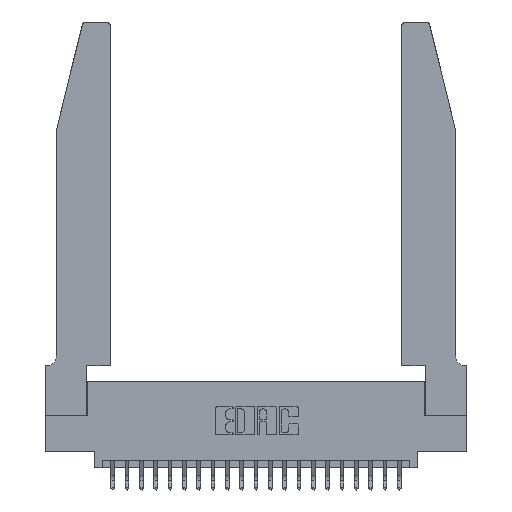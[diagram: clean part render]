
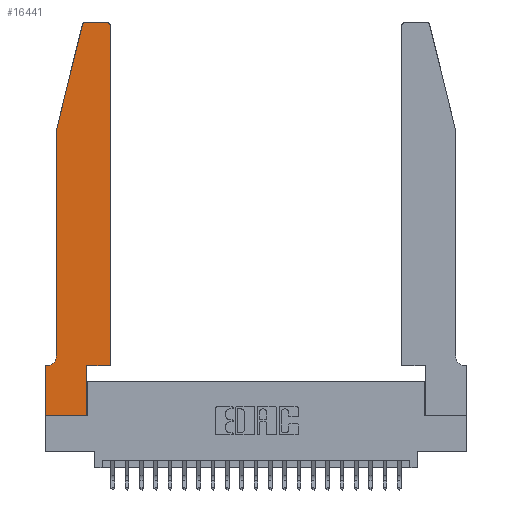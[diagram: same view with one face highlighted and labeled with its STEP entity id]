
A CAD part, top view. The second image highlights one B-rep face of the part: STEP entity #16441.
In plain terms, the highlighted planar face has unit normal (0, 0, 1).
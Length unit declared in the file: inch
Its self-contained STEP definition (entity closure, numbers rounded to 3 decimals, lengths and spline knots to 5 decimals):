
#87 = ORIENTED_EDGE ( 'NONE', *, *, #11937, .T. ) ;
#401 = CARTESIAN_POINT ( 'NONE',  ( 0.0755, 0.42, 0.37 ) ) ;
#807 = CARTESIAN_POINT ( 'NONE',  ( 0.4505, 2.72, 0.37 ) ) ;
#1071 = LINE ( 'NONE', #3253, #11936 ) ;
#1876 = EDGE_CURVE ( 'NONE', #4706, #23011, #15850, .T. ) ;
#1923 = LINE ( 'NONE', #15520, #8670 ) ;
#2167 = AXIS2_PLACEMENT_3D ( 'NONE', #2648, #19357, #4566 ) ;
#2179 = VECTOR ( 'NONE', #7909, 39.37008 ) ;
#2448 = VERTEX_POINT ( 'NONE', #6732 ) ;
#2648 = CARTESIAN_POINT ( 'NONE',  ( 0.284, 2.72, 0.37 ) ) ;
#3219 = CARTESIAN_POINT ( 'NONE',  ( 0.2865, 0.35, 0.37 ) ) ;
#3253 = CARTESIAN_POINT ( 'NONE',  ( 0.0755, 2., 0.37 ) ) ;
#3387 = ORIENTED_EDGE ( 'NONE', *, *, #3504, .T. ) ;
#3462 = CARTESIAN_POINT ( 'NONE',  ( 0., 0., 0.37 ) ) ;
#3504 = EDGE_CURVE ( 'NONE', #12758, #23851, #1071, .T. ) ;
#3602 = EDGE_CURVE ( 'NONE', #20908, #17066, #10462, .T. ) ;
#3861 = ORIENTED_EDGE ( 'NONE', *, *, #23042, .T. ) ;
#4566 = DIRECTION ( 'NONE',  ( 1., 0., 0. ) ) ;
#4706 = VERTEX_POINT ( 'NONE', #401 ) ;
#4806 = ORIENTED_EDGE ( 'NONE', *, *, #15787, .T. ) ;
#4998 = AXIS2_PLACEMENT_3D ( 'NONE', #20359, #10684, #22091 ) ;
#5570 = DIRECTION ( 'NONE',  ( 1., 0., 0. ) ) ;
#6584 = DIRECTION ( 'NONE',  ( -1., 0., 0. ) ) ;
#6600 = ORIENTED_EDGE ( 'NONE', *, *, #14183, .T. ) ;
#6732 = CARTESIAN_POINT ( 'NONE',  ( 0.2865, 0., 0.37 ) ) ;
#6839 = PLANE ( 'NONE',  #19540 ) ;
#6850 = DIRECTION ( 'NONE',  ( -0.239, -0.971, 0. ) ) ;
#6974 = EDGE_CURVE ( 'NONE', #17066, #8709, #1923, .T. ) ;
#7182 = FACE_OUTER_BOUND ( 'NONE', #18135, .T. ) ;
#7399 = DIRECTION ( 'NONE',  ( 1., 0., 0. ) ) ;
#7444 = ORIENTED_EDGE ( 'NONE', *, *, #20225, .T. ) ;
#7909 = DIRECTION ( 'NONE',  ( 0., -1., 0. ) ) ;
#8388 = LINE ( 'NONE', #22264, #13998 ) ;
#8462 = DIRECTION ( 'NONE',  ( 1., 0., 0. ) ) ;
#8602 = CARTESIAN_POINT ( 'NONE',  ( 0.2605, 2.75, 0.37 ) ) ;
#8670 = VECTOR ( 'NONE', #21132, 39.37008 ) ;
#8709 = VERTEX_POINT ( 'NONE', #807 ) ;
#8790 = ORIENTED_EDGE ( 'NONE', *, *, #3602, .T. ) ;
#8804 = LINE ( 'NONE', #15657, #22958 ) ;
#9231 = CARTESIAN_POINT ( 'NONE',  ( 0.25487, 2.72718, 0.37 ) ) ;
#9727 = CARTESIAN_POINT ( 'NONE',  ( 0., 0., 0.37 ) ) ;
#10190 = AXIS2_PLACEMENT_3D ( 'NONE', #14764, #15012, #5570 ) ;
#10255 = CARTESIAN_POINT ( 'NONE',  ( 0.0755, 0.35, 0.37 ) ) ;
#10462 = LINE ( 'NONE', #16329, #13725 ) ;
#10506 = CIRCLE ( 'NONE', #2167, 0.03 ) ;
#10563 = VERTEX_POINT ( 'NONE', #9727 ) ;
#10589 = CARTESIAN_POINT ( 'NONE',  ( 0., 0.35, 0.37 ) ) ;
#10609 = VECTOR ( 'NONE', #16385, 39.37008 ) ;
#10684 = DIRECTION ( 'NONE',  ( 0., 0., -1. ) ) ;
#10894 = LINE ( 'NONE', #3462, #10609 ) ;
#11936 = VECTOR ( 'NONE', #6850, 39.37008 ) ;
#11937 = EDGE_CURVE ( 'NONE', #21577, #15139, #20392, .T. ) ;
#12180 = DIRECTION ( 'NONE',  ( 0., 1., 0. ) ) ;
#12236 = DIRECTION ( 'NONE',  ( -1., 0., 0. ) ) ;
#12758 = VERTEX_POINT ( 'NONE', #9231 ) ;
#13725 = VECTOR ( 'NONE', #23914, 39.37008 ) ;
#13998 = VECTOR ( 'NONE', #7399, 39.37008 ) ;
#14183 = EDGE_CURVE ( 'NONE', #15139, #12758, #10506, .T. ) ;
#14686 = CARTESIAN_POINT ( 'NONE',  ( 0.284, 2.75, 0.37 ) ) ;
#14764 = CARTESIAN_POINT ( 'NONE',  ( 0.4205, 2.72, 0.37 ) ) ;
#15012 = DIRECTION ( 'NONE',  ( 0., 0., 1. ) ) ;
#15139 = VERTEX_POINT ( 'NONE', #14686 ) ;
#15520 = CARTESIAN_POINT ( 'NONE',  ( 0.4505, 0.35, 0.37 ) ) ;
#15657 = CARTESIAN_POINT ( 'NONE',  ( 0.2865, 0.35, 0.37 ) ) ;
#15787 = EDGE_CURVE ( 'NONE', #10563, #2448, #8388, .T. ) ;
#15850 = CIRCLE ( 'NONE', #4998, 0.07 ) ;
#16028 = EDGE_CURVE ( 'NONE', #8709, #21577, #21672, .T. ) ;
#16329 = CARTESIAN_POINT ( 'NONE',  ( 0.4505, 0.35, 0.37 ) ) ;
#16385 = DIRECTION ( 'NONE',  ( 0., -1., 0. ) ) ;
#16441 = ADVANCED_FACE ( 'NONE', ( #7182 ), #6839, .T. ) ;
#17066 = VERTEX_POINT ( 'NONE', #23206 ) ;
#17149 = CARTESIAN_POINT ( 'NONE',  ( 0.0755, 2., 0.37 ) ) ;
#17191 = LINE ( 'NONE', #17248, #2179 ) ;
#17248 = CARTESIAN_POINT ( 'NONE',  ( 0.0755, 2., 0.37 ) ) ;
#17677 = EDGE_CURVE ( 'NONE', #23851, #4706, #17191, .T. ) ;
#18135 = EDGE_LOOP ( 'NONE', ( #87, #6600, #3387, #18220, #24267, #3861, #20134, #4806, #7444, #8790, #19129, #21297 ) ) ;
#18220 = ORIENTED_EDGE ( 'NONE', *, *, #17677, .T. ) ;
#18991 = VECTOR ( 'NONE', #12236, 39.37008 ) ;
#19105 = EDGE_CURVE ( 'NONE', #23397, #10563, #10894, .T. ) ;
#19129 = ORIENTED_EDGE ( 'NONE', *, *, #6974, .T. ) ;
#19357 = DIRECTION ( 'NONE',  ( 0., 0., 1. ) ) ;
#19540 = AXIS2_PLACEMENT_3D ( 'NONE', #10589, #23741, #8462 ) ;
#20134 = ORIENTED_EDGE ( 'NONE', *, *, #19105, .T. ) ;
#20225 = EDGE_CURVE ( 'NONE', #2448, #20908, #8804, .T. ) ;
#20359 = CARTESIAN_POINT ( 'NONE',  ( 0.0055, 0.42, 0.37 ) ) ;
#20392 = LINE ( 'NONE', #8602, #22453 ) ;
#20518 = CARTESIAN_POINT ( 'NONE',  ( 0.0055, 0.35, 0.37 ) ) ;
#20908 = VERTEX_POINT ( 'NONE', #3219 ) ;
#21132 = DIRECTION ( 'NONE',  ( 0., 1., 0. ) ) ;
#21297 = ORIENTED_EDGE ( 'NONE', *, *, #16028, .T. ) ;
#21577 = VERTEX_POINT ( 'NONE', #23944 ) ;
#21672 = CIRCLE ( 'NONE', #10190, 0.03 ) ;
#22091 = DIRECTION ( 'NONE',  ( -1., 0., 0. ) ) ;
#22264 = CARTESIAN_POINT ( 'NONE',  ( 0., 0., 0.37 ) ) ;
#22453 = VECTOR ( 'NONE', #6584, 39.37008 ) ;
#22712 = CARTESIAN_POINT ( 'NONE',  ( 0., 0.35, 0.37 ) ) ;
#22958 = VECTOR ( 'NONE', #12180, 39.37008 ) ;
#23011 = VERTEX_POINT ( 'NONE', #20518 ) ;
#23042 = EDGE_CURVE ( 'NONE', #23011, #23397, #24025, .T. ) ;
#23206 = CARTESIAN_POINT ( 'NONE',  ( 0.4505, 0.35, 0.37 ) ) ;
#23397 = VERTEX_POINT ( 'NONE', #22712 ) ;
#23741 = DIRECTION ( 'NONE',  ( 0., 0., 1. ) ) ;
#23851 = VERTEX_POINT ( 'NONE', #17149 ) ;
#23914 = DIRECTION ( 'NONE',  ( 1., 0., 0. ) ) ;
#23944 = CARTESIAN_POINT ( 'NONE',  ( 0.4205, 2.75, 0.37 ) ) ;
#24025 = LINE ( 'NONE', #10255, #18991 ) ;
#24267 = ORIENTED_EDGE ( 'NONE', *, *, #1876, .T. ) ;
